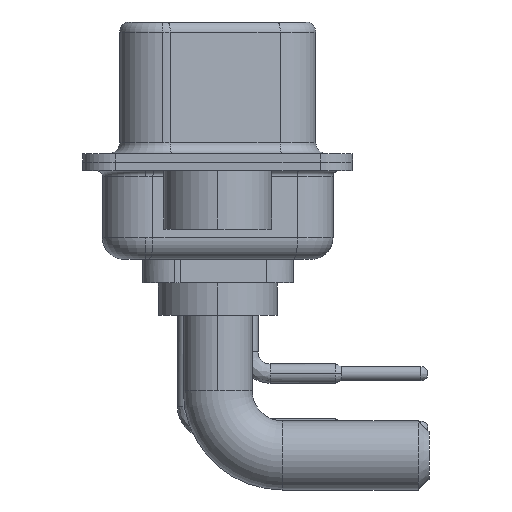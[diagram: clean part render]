
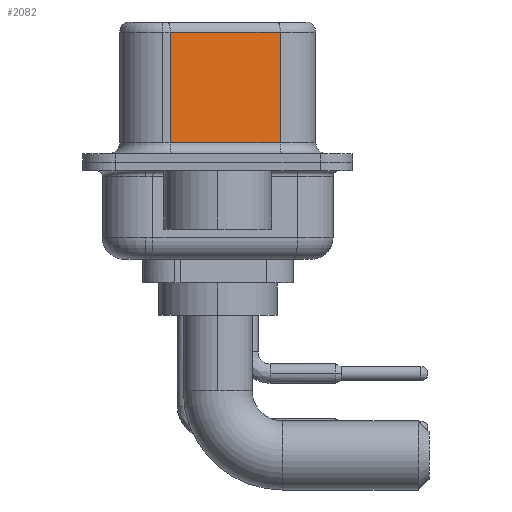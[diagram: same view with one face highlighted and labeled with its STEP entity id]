
A CAD part, left-side view. The second image highlights one B-rep face of the part: STEP entity #2082.
In plain terms, the highlighted planar face has unit normal (-0.985, -0.174, 0).
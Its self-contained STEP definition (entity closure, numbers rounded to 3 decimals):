
#97 = DIRECTION ( 'NONE',  ( 0., 0., -1. ) ) ;
#521 = ORIENTED_EDGE ( 'NONE', *, *, #4328, .F. ) ;
#1412 = LINE ( 'NONE', #16677, #2596 ) ;
#1730 = VECTOR ( 'NONE', #20558, 1000. ) ;
#2082 = ADVANCED_FACE ( 'NONE', ( #12811 ), #12446, .F. ) ;
#2596 = VECTOR ( 'NONE', #22422, 1000. ) ;
#3452 = DIRECTION ( 'NONE',  ( -0.174, 0.985, 0. ) ) ;
#4328 = EDGE_CURVE ( 'NONE', #17394, #14161, #5589, .T. ) ;
#4643 = EDGE_CURVE ( 'NONE', #17394, #9742, #18359, .T. ) ;
#5273 = VECTOR ( 'NONE', #3452, 1000. ) ;
#5589 = LINE ( 'NONE', #23257, #12077 ) ;
#7964 = VERTEX_POINT ( 'NONE', #8726 ) ;
#8006 = CARTESIAN_POINT ( 'NONE',  ( 3.68, 2.203, 6.02 ) ) ;
#8726 = CARTESIAN_POINT ( 'NONE',  ( 3.68, 2.203, 0.9 ) ) ;
#9070 = EDGE_CURVE ( 'NONE', #7964, #14161, #1412, .T. ) ;
#9742 = VERTEX_POINT ( 'NONE', #8006 ) ;
#10900 = LINE ( 'NONE', #13045, #1730 ) ;
#12077 = VECTOR ( 'NONE', #97, 1000. ) ;
#12446 = PLANE ( 'NONE',  #14975 ) ;
#12768 = ORIENTED_EDGE ( 'NONE', *, *, #9070, .T. ) ;
#12811 = FACE_OUTER_BOUND ( 'NONE', #20220, .T. ) ;
#12877 = ORIENTED_EDGE ( 'NONE', *, *, #4643, .T. ) ;
#13045 = CARTESIAN_POINT ( 'NONE',  ( 3.68, 2.203, 6.52 ) ) ;
#14161 = VERTEX_POINT ( 'NONE', #24484 ) ;
#14975 = AXIS2_PLACEMENT_3D ( 'NONE', #24356, #20326, #20087 ) ;
#16677 = CARTESIAN_POINT ( 'NONE',  ( 4.58, -2.897, 0.9 ) ) ;
#16727 = CARTESIAN_POINT ( 'NONE',  ( 4.58, -2.897, 6.02 ) ) ;
#17149 = ORIENTED_EDGE ( 'NONE', *, *, #24536, .T. ) ;
#17394 = VERTEX_POINT ( 'NONE', #16727 ) ;
#18359 = LINE ( 'NONE', #18482, #5273 ) ;
#18482 = CARTESIAN_POINT ( 'NONE',  ( 4.58, -2.897, 6.02 ) ) ;
#20087 = DIRECTION ( 'NONE',  ( -0.174, 0.985, 0. ) ) ;
#20220 = EDGE_LOOP ( 'NONE', ( #521, #12877, #17149, #12768 ) ) ;
#20326 = DIRECTION ( 'NONE',  ( 0.985, 0.174, 0. ) ) ;
#20558 = DIRECTION ( 'NONE',  ( 0., 0., -1. ) ) ;
#22422 = DIRECTION ( 'NONE',  ( 0.174, -0.985, 0. ) ) ;
#23257 = CARTESIAN_POINT ( 'NONE',  ( 4.58, -2.897, 6.52 ) ) ;
#24356 = CARTESIAN_POINT ( 'NONE',  ( 4.58, -2.897, 6.52 ) ) ;
#24484 = CARTESIAN_POINT ( 'NONE',  ( 4.58, -2.897, 0.9 ) ) ;
#24536 = EDGE_CURVE ( 'NONE', #9742, #7964, #10900, .T. ) ;
